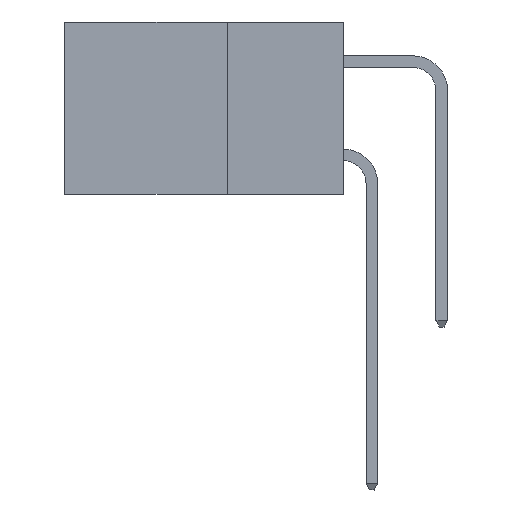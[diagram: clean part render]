
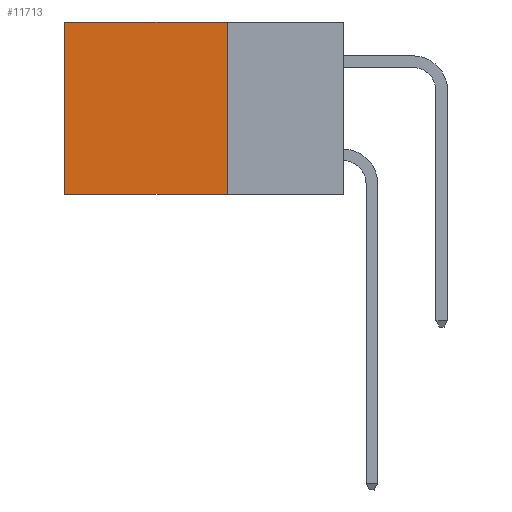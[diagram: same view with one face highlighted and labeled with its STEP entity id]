
A CAD part, left-side view. The second image highlights one B-rep face of the part: STEP entity #11713.
In plain terms, the highlighted planar face has unit normal (-1, 0, 0).
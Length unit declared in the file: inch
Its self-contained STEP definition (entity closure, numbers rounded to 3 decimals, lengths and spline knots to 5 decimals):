
#1426 = VERTEX_POINT ( 'NONE', #22819 ) ;
#2678 = CARTESIAN_POINT ( 'NONE',  ( 0.298, 0.25, 0. ) ) ;
#2796 = CARTESIAN_POINT ( 'NONE',  ( 0.298, 0.25, 0. ) ) ;
#3895 = CARTESIAN_POINT ( 'NONE',  ( 0.298, 0.25, -0.37 ) ) ;
#5250 = LINE ( 'NONE', #3895, #24401 ) ;
#5313 = PLANE ( 'NONE',  #20625 ) ;
#5421 = EDGE_CURVE ( 'NONE', #14552, #1426, #23101, .T. ) ;
#6413 = ORIENTED_EDGE ( 'NONE', *, *, #16317, .T. ) ;
#6786 = DIRECTION ( 'NONE',  ( 0., 1., 0. ) ) ;
#7609 = EDGE_CURVE ( 'NONE', #14552, #30488, #18041, .T. ) ;
#7699 = ORIENTED_EDGE ( 'NONE', *, *, #5421, .T. ) ;
#9857 = VECTOR ( 'NONE', #6786, 39.37008 ) ;
#10205 = LINE ( 'NONE', #32136, #23442 ) ;
#10436 = DIRECTION ( 'NONE',  ( 0., 0., -1. ) ) ;
#10463 = DIRECTION ( 'NONE',  ( 0., 0., -1. ) ) ;
#10970 = ORIENTED_EDGE ( 'NONE', *, *, #13208, .F. ) ;
#11713 = ADVANCED_FACE ( 'NONE', ( #28186 ), #5313, .F. ) ;
#13208 = EDGE_CURVE ( 'NONE', #30488, #19886, #5250, .T. ) ;
#14552 = VERTEX_POINT ( 'NONE', #2678 ) ;
#15073 = ORIENTED_EDGE ( 'NONE', *, *, #7609, .F. ) ;
#16317 = EDGE_CURVE ( 'NONE', #1426, #19886, #10205, .T. ) ;
#17259 = VECTOR ( 'NONE', #10463, 39.37008 ) ;
#17340 = DIRECTION ( 'NONE',  ( 0., 0., -1. ) ) ;
#18041 = LINE ( 'NONE', #2796, #17259 ) ;
#19270 = CARTESIAN_POINT ( 'NONE',  ( 0.298, 0.25, 0. ) ) ;
#19886 = VERTEX_POINT ( 'NONE', #20405 ) ;
#20405 = CARTESIAN_POINT ( 'NONE',  ( 0.298, 0.6, -0.37 ) ) ;
#20625 = AXIS2_PLACEMENT_3D ( 'NONE', #22823, #25293, #10436 ) ;
#21425 = DIRECTION ( 'NONE',  ( 0., 1., 0. ) ) ;
#22819 = CARTESIAN_POINT ( 'NONE',  ( 0.298, 0.6, 0. ) ) ;
#22823 = CARTESIAN_POINT ( 'NONE',  ( 0.298, 0.25, 0. ) ) ;
#23089 = CARTESIAN_POINT ( 'NONE',  ( 0.298, 0.25, -0.37 ) ) ;
#23101 = LINE ( 'NONE', #19270, #9857 ) ;
#23442 = VECTOR ( 'NONE', #17340, 39.37008 ) ;
#24401 = VECTOR ( 'NONE', #21425, 39.37008 ) ;
#25293 = DIRECTION ( 'NONE',  ( 1., 0., 0. ) ) ;
#26900 = EDGE_LOOP ( 'NONE', ( #6413, #10970, #15073, #7699 ) ) ;
#28186 = FACE_OUTER_BOUND ( 'NONE', #26900, .T. ) ;
#30488 = VERTEX_POINT ( 'NONE', #23089 ) ;
#32136 = CARTESIAN_POINT ( 'NONE',  ( 0.298, 0.6, 0. ) ) ;
